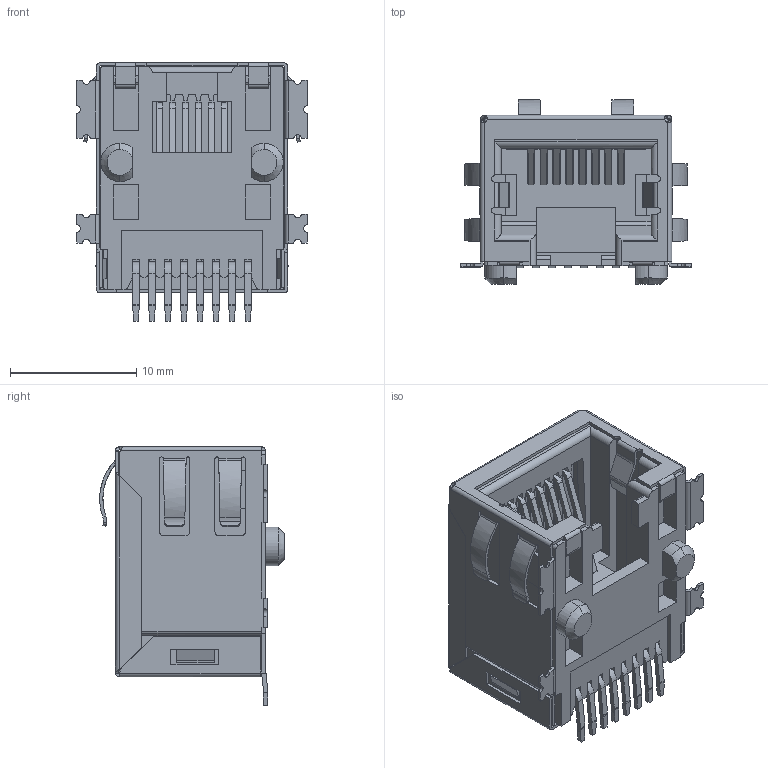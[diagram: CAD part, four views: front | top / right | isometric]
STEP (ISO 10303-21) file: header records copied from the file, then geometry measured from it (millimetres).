
FILE_DESCRIPTION (( 'STEP AP203' ), '1' );
FILE_NAME ('RJS8018824L00202.STEP', '2020-02-03T15:27:27', ( '' ), ( '' ), 'SwSTEP 2.0', 'SolidWorks 2016', '' );
FILE_SCHEMA (( 'CONFIG_CONTROL_DESIGN' ));
Length unit declared in the file: millimetre
Products named in the file (4): S8 Contacts; S8 Insulator; RJS8018824L00202; S8 Shield
Assembly tree (3 placements, depth 2):
  RJS8018824L00202
    S8 Insulator
    S8 Contacts
    S8 Shield
Bounding box: 18.3 x 14.65 x 20.5 mm (x, y, z)
Volume: 1308.3 mm3; surface area: 4634.3 mm2
Topology: 10 solids, 10 shells, 976 faces, 2713 edges, 1753 vertices
Faces by surface type: plane 602, cylinder 314, bspline 54, cone 6
Entity records: 33484 total; most frequent: CARTESIAN_POINT 8309, ORIENTED_EDGE 5426, DIRECTION 4834, EDGE_CURVE 2713, LINE 1924, VECTOR 1924, VERTEX_POINT 1753, AXIS2_PLACEMENT_3D 1455
